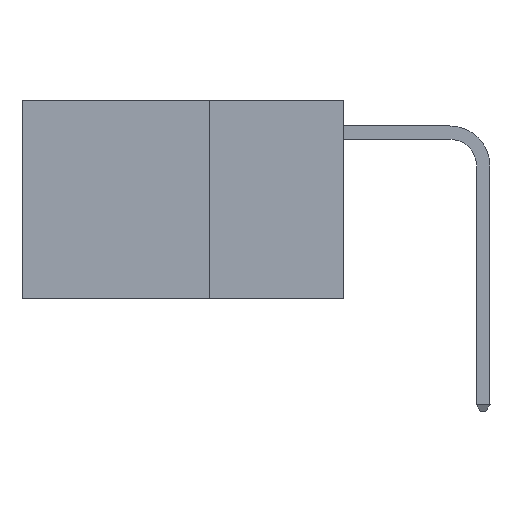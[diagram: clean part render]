
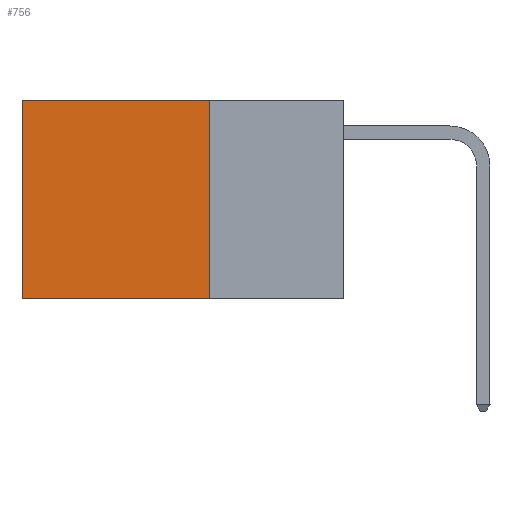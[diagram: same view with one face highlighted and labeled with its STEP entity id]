
A CAD part, left-side view. The second image highlights one B-rep face of the part: STEP entity #756.
In plain terms, the highlighted planar face has unit normal (-1, 0, 0).
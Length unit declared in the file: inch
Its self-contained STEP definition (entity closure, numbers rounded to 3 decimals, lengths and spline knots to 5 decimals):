
#3 = CARTESIAN_POINT ( 'NONE',  ( 0.2625, 0.25, 0. ) ) ;
#391 = DIRECTION ( 'NONE',  ( 0., 0., -1. ) ) ;
#558 = VERTEX_POINT ( 'NONE', #7648 ) ;
#638 = EDGE_CURVE ( 'NONE', #1291, #558, #771, .T. ) ;
#756 = ADVANCED_FACE ( 'NONE', ( #7533 ), #5530, .F. ) ;
#771 = LINE ( 'NONE', #2446, #3080 ) ;
#823 = VECTOR ( 'NONE', #391, 39.37008 ) ;
#1085 = EDGE_CURVE ( 'NONE', #558, #6529, #3540, .T. ) ;
#1291 = VERTEX_POINT ( 'NONE', #3 ) ;
#2084 = ORIENTED_EDGE ( 'NONE', *, *, #7524, .F. ) ;
#2446 = CARTESIAN_POINT ( 'NONE',  ( 0.2625, 0.25, 0. ) ) ;
#2492 = CARTESIAN_POINT ( 'NONE',  ( 0.2625, 0.25, -0.37 ) ) ;
#2715 = CARTESIAN_POINT ( 'NONE',  ( 0.2625, 0.25, 0. ) ) ;
#3080 = VECTOR ( 'NONE', #5368, 39.37008 ) ;
#3540 = LINE ( 'NONE', #6372, #5369 ) ;
#3612 = ORIENTED_EDGE ( 'NONE', *, *, #9199, .F. ) ;
#3687 = VECTOR ( 'NONE', #7169, 39.37008 ) ;
#4814 = DIRECTION ( 'NONE',  ( 1., 0., 0. ) ) ;
#5073 = DIRECTION ( 'NONE',  ( 0., 0., -1. ) ) ;
#5368 = DIRECTION ( 'NONE',  ( 0., 1., 0. ) ) ;
#5369 = VECTOR ( 'NONE', #5073, 39.37008 ) ;
#5530 = PLANE ( 'NONE',  #7408 ) ;
#5607 = CARTESIAN_POINT ( 'NONE',  ( 0.2625, 0.25, -0.37 ) ) ;
#6372 = CARTESIAN_POINT ( 'NONE',  ( 0.2625, 0.6, 0. ) ) ;
#6529 = VERTEX_POINT ( 'NONE', #9248 ) ;
#7169 = DIRECTION ( 'NONE',  ( 0., 1., 0. ) ) ;
#7408 = AXIS2_PLACEMENT_3D ( 'NONE', #2715, #4814, #9386 ) ;
#7521 = ORIENTED_EDGE ( 'NONE', *, *, #1085, .T. ) ;
#7524 = EDGE_CURVE ( 'NONE', #9478, #6529, #9311, .T. ) ;
#7533 = FACE_OUTER_BOUND ( 'NONE', #8589, .T. ) ;
#7648 = CARTESIAN_POINT ( 'NONE',  ( 0.2625, 0.6, 0. ) ) ;
#7778 = CARTESIAN_POINT ( 'NONE',  ( 0.2625, 0.25, 0. ) ) ;
#7958 = LINE ( 'NONE', #7778, #823 ) ;
#8385 = ORIENTED_EDGE ( 'NONE', *, *, #638, .T. ) ;
#8589 = EDGE_LOOP ( 'NONE', ( #7521, #2084, #3612, #8385 ) ) ;
#9199 = EDGE_CURVE ( 'NONE', #1291, #9478, #7958, .T. ) ;
#9248 = CARTESIAN_POINT ( 'NONE',  ( 0.2625, 0.6, -0.37 ) ) ;
#9311 = LINE ( 'NONE', #5607, #3687 ) ;
#9386 = DIRECTION ( 'NONE',  ( 0., 0., -1. ) ) ;
#9478 = VERTEX_POINT ( 'NONE', #2492 ) ;
